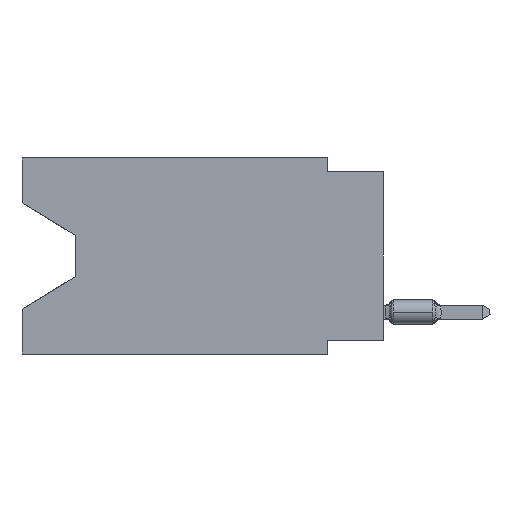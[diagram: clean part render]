
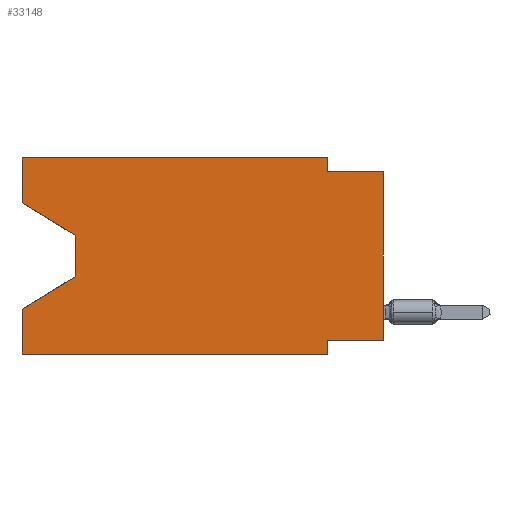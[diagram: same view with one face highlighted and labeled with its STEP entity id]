
A CAD part, left-side view. The second image highlights one B-rep face of the part: STEP entity #33148.
In plain terms, the highlighted planar face has unit normal (-1, 0, 0).
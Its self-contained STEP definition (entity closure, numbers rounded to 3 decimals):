
#41 = VECTOR ( 'NONE', #21048, 1000. ) ;
#548 = DIRECTION ( 'NONE',  ( 0., -1., 0. ) ) ;
#2139 = CARTESIAN_POINT ( 'NONE',  ( 0., 16.383, 0. ) ) ;
#2473 = CARTESIAN_POINT ( 'NONE',  ( 0., 2.54, -8.89 ) ) ;
#2881 = VECTOR ( 'NONE', #20976, 1000. ) ;
#3057 = VERTEX_POINT ( 'NONE', #2473 ) ;
#3206 = VECTOR ( 'NONE', #48375, 1000. ) ;
#3634 = EDGE_CURVE ( 'NONE', #28386, #48472, #5129, .T. ) ;
#4022 = ORIENTED_EDGE ( 'NONE', *, *, #18450, .T. ) ;
#4282 = CARTESIAN_POINT ( 'NONE',  ( 0., 0., 0. ) ) ;
#4715 = EDGE_CURVE ( 'NONE', #33350, #28386, #47843, .T. ) ;
#4750 = ORIENTED_EDGE ( 'NONE', *, *, #33565, .F. ) ;
#4925 = LINE ( 'NONE', #46664, #5263 ) ;
#5129 = LINE ( 'NONE', #43611, #2881 ) ;
#5226 = VECTOR ( 'NONE', #36966, 1000. ) ;
#5263 = VECTOR ( 'NONE', #20502, 1000. ) ;
#5639 = DIRECTION ( 'NONE',  ( 0., 0., -1. ) ) ;
#6246 = CARTESIAN_POINT ( 'NONE',  ( 0., 16.383, 0. ) ) ;
#6282 = VERTEX_POINT ( 'NONE', #38319 ) ;
#6347 = PLANE ( 'NONE',  #48244 ) ;
#6591 = FACE_OUTER_BOUND ( 'NONE', #41928, .T. ) ;
#7439 = CARTESIAN_POINT ( 'NONE',  ( 0., 0., -0.635 ) ) ;
#7450 = LINE ( 'NONE', #21155, #15330 ) ;
#7776 = DIRECTION ( 'NONE',  ( 0., 0., 1. ) ) ;
#8295 = DIRECTION ( 'NONE',  ( 0., 0.855, -0.519 ) ) ;
#9935 = DIRECTION ( 'NONE',  ( 0., -1., 0. ) ) ;
#10094 = CARTESIAN_POINT ( 'NONE',  ( 0., 16.383, -2.038 ) ) ;
#10354 = EDGE_CURVE ( 'NONE', #48089, #3057, #11317, .T. ) ;
#11083 = CARTESIAN_POINT ( 'NONE',  ( 0., 16.383, -2.038 ) ) ;
#11317 = LINE ( 'NONE', #26681, #44785 ) ;
#12067 = CARTESIAN_POINT ( 'NONE',  ( 0., 13.97, -5.385 ) ) ;
#12242 = CARTESIAN_POINT ( 'NONE',  ( 0., 2.54, -8.89 ) ) ;
#14112 = EDGE_CURVE ( 'NONE', #48089, #44929, #32796, .T. ) ;
#14119 = VERTEX_POINT ( 'NONE', #25491 ) ;
#14374 = DIRECTION ( 'NONE',  ( 0., 0., -1. ) ) ;
#15330 = VECTOR ( 'NONE', #22803, 1000. ) ;
#15991 = ORIENTED_EDGE ( 'NONE', *, *, #4715, .T. ) ;
#16625 = CARTESIAN_POINT ( 'NONE',  ( 0., 13.97, -5.385 ) ) ;
#17494 = LINE ( 'NONE', #40889, #28698 ) ;
#17878 = EDGE_CURVE ( 'NONE', #33350, #42300, #43177, .T. ) ;
#18450 = EDGE_CURVE ( 'NONE', #48472, #44929, #20364, .T. ) ;
#20364 = LINE ( 'NONE', #12067, #30494 ) ;
#20502 = DIRECTION ( 'NONE',  ( 0., 0., -1. ) ) ;
#20793 = CARTESIAN_POINT ( 'NONE',  ( 0., 2.54, -8.255 ) ) ;
#20976 = DIRECTION ( 'NONE',  ( 0., 0., -1. ) ) ;
#21048 = DIRECTION ( 'NONE',  ( 0., 0., 1. ) ) ;
#21155 = CARTESIAN_POINT ( 'NONE',  ( 0., 0., -8.255 ) ) ;
#21226 = CARTESIAN_POINT ( 'NONE',  ( 0., 16.383, -8.89 ) ) ;
#22803 = DIRECTION ( 'NONE',  ( 0., 1., 0. ) ) ;
#23349 = EDGE_CURVE ( 'NONE', #14119, #29447, #34443, .T. ) ;
#24804 = CARTESIAN_POINT ( 'NONE',  ( 0., 16.383, 0. ) ) ;
#25318 = CARTESIAN_POINT ( 'NONE',  ( 0., 16.383, -6.852 ) ) ;
#25491 = CARTESIAN_POINT ( 'NONE',  ( 0., 0., -8.255 ) ) ;
#25709 = DIRECTION ( 'NONE',  ( 0., -0.855, -0.519 ) ) ;
#25944 = VECTOR ( 'NONE', #5639, 1000. ) ;
#26681 = CARTESIAN_POINT ( 'NONE',  ( 0., 16.383, -8.89 ) ) ;
#26832 = CARTESIAN_POINT ( 'NONE',  ( 0., 13.97, -3.505 ) ) ;
#28085 = ORIENTED_EDGE ( 'NONE', *, *, #14112, .F. ) ;
#28124 = ORIENTED_EDGE ( 'NONE', *, *, #35575, .F. ) ;
#28386 = VERTEX_POINT ( 'NONE', #26832 ) ;
#28698 = VECTOR ( 'NONE', #9935, 1000. ) ;
#29194 = ORIENTED_EDGE ( 'NONE', *, *, #49192, .F. ) ;
#29447 = VERTEX_POINT ( 'NONE', #7439 ) ;
#30494 = VECTOR ( 'NONE', #8295, 1000. ) ;
#31724 = ORIENTED_EDGE ( 'NONE', *, *, #23349, .T. ) ;
#31981 = VERTEX_POINT ( 'NONE', #34139 ) ;
#32761 = CARTESIAN_POINT ( 'NONE',  ( 0., 16.383, 0. ) ) ;
#32796 = LINE ( 'NONE', #2139, #3206 ) ;
#33010 = DIRECTION ( 'NONE',  ( 1., 0., 0. ) ) ;
#33148 = ADVANCED_FACE ( 'NONE', ( #6591 ), #6347, .F. ) ;
#33350 = VERTEX_POINT ( 'NONE', #11083 ) ;
#33407 = LINE ( 'NONE', #46166, #5226 ) ;
#33565 = EDGE_CURVE ( 'NONE', #14119, #41268, #7450, .T. ) ;
#34139 = CARTESIAN_POINT ( 'NONE',  ( 0., 2.54, 0. ) ) ;
#34443 = LINE ( 'NONE', #4282, #45850 ) ;
#35575 = EDGE_CURVE ( 'NONE', #41268, #3057, #40099, .T. ) ;
#36966 = DIRECTION ( 'NONE',  ( 0., -1., 0. ) ) ;
#38039 = EDGE_CURVE ( 'NONE', #6282, #29447, #33407, .T. ) ;
#38053 = ORIENTED_EDGE ( 'NONE', *, *, #10354, .T. ) ;
#38248 = EDGE_CURVE ( 'NONE', #31981, #6282, #4925, .T. ) ;
#38319 = CARTESIAN_POINT ( 'NONE',  ( 0., 2.54, -0.635 ) ) ;
#39118 = VECTOR ( 'NONE', #25709, 1000. ) ;
#39876 = ORIENTED_EDGE ( 'NONE', *, *, #17878, .F. ) ;
#40099 = LINE ( 'NONE', #12242, #25944 ) ;
#40889 = CARTESIAN_POINT ( 'NONE',  ( 0., 16.383, 0. ) ) ;
#41268 = VERTEX_POINT ( 'NONE', #20793 ) ;
#41928 = EDGE_LOOP ( 'NONE', ( #15991, #49354, #4022, #28085, #38053, #28124, #4750, #31724, #49328, #47711, #29194, #39876 ) ) ;
#42300 = VERTEX_POINT ( 'NONE', #6246 ) ;
#43177 = LINE ( 'NONE', #24804, #41 ) ;
#43611 = CARTESIAN_POINT ( 'NONE',  ( 0., 13.97, -3.505 ) ) ;
#44785 = VECTOR ( 'NONE', #548, 1000. ) ;
#44929 = VERTEX_POINT ( 'NONE', #25318 ) ;
#45850 = VECTOR ( 'NONE', #7776, 1000. ) ;
#46166 = CARTESIAN_POINT ( 'NONE',  ( 0., 0., -0.635 ) ) ;
#46664 = CARTESIAN_POINT ( 'NONE',  ( 0., 2.54, 0. ) ) ;
#47711 = ORIENTED_EDGE ( 'NONE', *, *, #38248, .F. ) ;
#47843 = LINE ( 'NONE', #10094, #39118 ) ;
#48089 = VERTEX_POINT ( 'NONE', #21226 ) ;
#48244 = AXIS2_PLACEMENT_3D ( 'NONE', #32761, #33010, #14374 ) ;
#48375 = DIRECTION ( 'NONE',  ( 0., 0., 1. ) ) ;
#48472 = VERTEX_POINT ( 'NONE', #16625 ) ;
#49192 = EDGE_CURVE ( 'NONE', #42300, #31981, #17494, .T. ) ;
#49328 = ORIENTED_EDGE ( 'NONE', *, *, #38039, .F. ) ;
#49354 = ORIENTED_EDGE ( 'NONE', *, *, #3634, .T. ) ;
